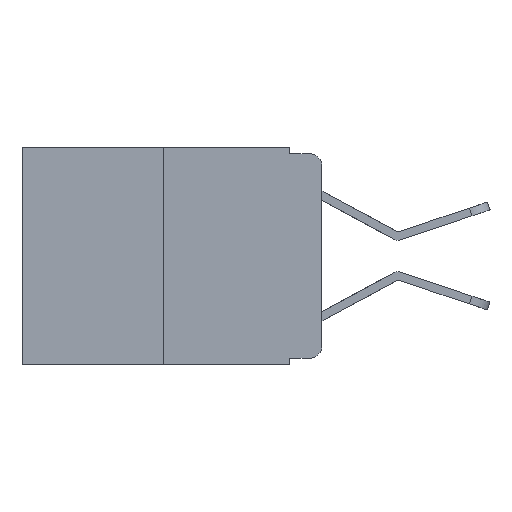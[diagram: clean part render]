
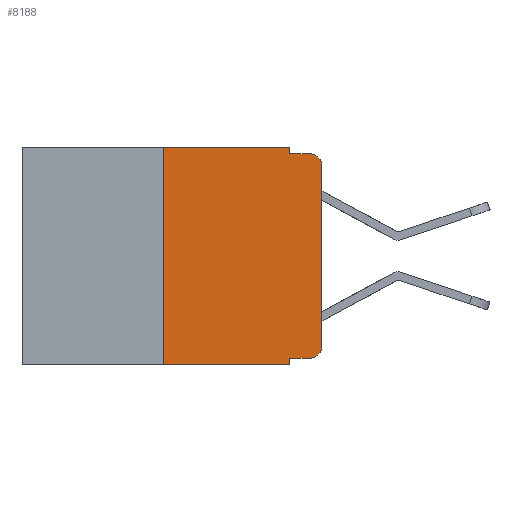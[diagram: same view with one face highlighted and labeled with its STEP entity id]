
A CAD part, left-side view. The second image highlights one B-rep face of the part: STEP entity #8188.
In plain terms, the highlighted planar face has unit normal (-1, 0, 0).
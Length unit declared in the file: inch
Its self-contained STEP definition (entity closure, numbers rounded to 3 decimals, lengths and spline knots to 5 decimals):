
#37 = EDGE_CURVE ( 'NONE', #5727, #10715, #5399, .T. ) ;
#81 = DIRECTION ( 'NONE',  ( 0., -1., 0. ) ) ;
#416 = CARTESIAN_POINT ( 'NONE',  ( 0., 0.02, -0.01 ) ) ;
#569 = CARTESIAN_POINT ( 'NONE',  ( 0., 0., -0.313 ) ) ;
#613 = DIRECTION ( 'NONE',  ( 0., 0., -1. ) ) ;
#999 = ORIENTED_EDGE ( 'NONE', *, *, #1486, .F. ) ;
#1174 = CARTESIAN_POINT ( 'NONE',  ( 0., 0.051, 0. ) ) ;
#1313 = VECTOR ( 'NONE', #13324, 39.37008 ) ;
#1486 = EDGE_CURVE ( 'NONE', #10284, #11984, #14424, .T. ) ;
#1920 = VERTEX_POINT ( 'NONE', #12047 ) ;
#1991 = DIRECTION ( 'NONE',  ( 1., 0., 0. ) ) ;
#2308 = EDGE_CURVE ( 'NONE', #11984, #10111, #4769, .T. ) ;
#2555 = VECTOR ( 'NONE', #4273, 39.37008 ) ;
#2671 = DIRECTION ( 'NONE',  ( 0., -1., 0. ) ) ;
#2691 = CIRCLE ( 'NONE', #7017, 0.02 ) ;
#3013 = VECTOR ( 'NONE', #9646, 39.37008 ) ;
#3077 = VECTOR ( 'NONE', #2671, 39.37008 ) ;
#3184 = LINE ( 'NONE', #7799, #3722 ) ;
#3427 = ORIENTED_EDGE ( 'NONE', *, *, #11608, .T. ) ;
#3722 = VECTOR ( 'NONE', #81, 39.37008 ) ;
#3765 = ORIENTED_EDGE ( 'NONE', *, *, #12278, .F. ) ;
#3883 = CARTESIAN_POINT ( 'NONE',  ( 0., 0.25, 0. ) ) ;
#4033 = ORIENTED_EDGE ( 'NONE', *, *, #2308, .F. ) ;
#4186 = ORIENTED_EDGE ( 'NONE', *, *, #12717, .F. ) ;
#4271 = CARTESIAN_POINT ( 'NONE',  ( 0., 0.25, 0. ) ) ;
#4273 = DIRECTION ( 'NONE',  ( 0., 0., -1. ) ) ;
#4377 = ORIENTED_EDGE ( 'NONE', *, *, #7946, .T. ) ;
#4607 = VERTEX_POINT ( 'NONE', #11918 ) ;
#4769 = LINE ( 'NONE', #9403, #3077 ) ;
#5012 = VECTOR ( 'NONE', #12851, 39.37008 ) ;
#5063 = DIRECTION ( 'NONE',  ( -1., 0., 0. ) ) ;
#5078 = LINE ( 'NONE', #3883, #3013 ) ;
#5274 = CARTESIAN_POINT ( 'NONE',  ( 0., 0., -0.03 ) ) ;
#5308 = LINE ( 'NONE', #11133, #1313 ) ;
#5399 = LINE ( 'NONE', #12344, #5012 ) ;
#5539 = CARTESIAN_POINT ( 'NONE',  ( 0., 0.473, 0. ) ) ;
#5700 = CIRCLE ( 'NONE', #13659, 0.02 ) ;
#5727 = VERTEX_POINT ( 'NONE', #569 ) ;
#6055 = CARTESIAN_POINT ( 'NONE',  ( 0., 0.25, -0.343 ) ) ;
#6186 = AXIS2_PLACEMENT_3D ( 'NONE', #5539, #1991, #11215 ) ;
#6683 = ORIENTED_EDGE ( 'NONE', *, *, #37, .T. ) ;
#6696 = DIRECTION ( 'NONE',  ( 0., 0., -1. ) ) ;
#6735 = VERTEX_POINT ( 'NONE', #4271 ) ;
#6973 = ORIENTED_EDGE ( 'NONE', *, *, #9064, .T. ) ;
#7017 = AXIS2_PLACEMENT_3D ( 'NONE', #9837, #5063, #613 ) ;
#7126 = VECTOR ( 'NONE', #9955, 39.37008 ) ;
#7762 = FACE_OUTER_BOUND ( 'NONE', #10482, .T. ) ;
#7799 = CARTESIAN_POINT ( 'NONE',  ( 0., 0.473, -0.343 ) ) ;
#7946 = EDGE_CURVE ( 'NONE', #10715, #10111, #2691, .T. ) ;
#7966 = CARTESIAN_POINT ( 'NONE',  ( 0., 0.02, -0.313 ) ) ;
#8121 = VECTOR ( 'NONE', #6696, 39.37008 ) ;
#8188 = ADVANCED_FACE ( 'NONE', ( #7762 ), #12337, .F. ) ;
#8702 = CARTESIAN_POINT ( 'NONE',  ( 0., 0.473, 0. ) ) ;
#8847 = VERTEX_POINT ( 'NONE', #6055 ) ;
#9012 = CARTESIAN_POINT ( 'NONE',  ( 0., 0.051, 0. ) ) ;
#9064 = EDGE_CURVE ( 'NONE', #8847, #4607, #3184, .T. ) ;
#9403 = CARTESIAN_POINT ( 'NONE',  ( 0., 0.051, -0.01 ) ) ;
#9457 = VERTEX_POINT ( 'NONE', #9904 ) ;
#9646 = DIRECTION ( 'NONE',  ( 0., 0., 1. ) ) ;
#9837 = CARTESIAN_POINT ( 'NONE',  ( 0., 0.02, -0.03 ) ) ;
#9904 = CARTESIAN_POINT ( 'NONE',  ( 0., 0.051, -0.333 ) ) ;
#9955 = DIRECTION ( 'NONE',  ( 0., -1., 0. ) ) ;
#10111 = VERTEX_POINT ( 'NONE', #416 ) ;
#10284 = VERTEX_POINT ( 'NONE', #9012 ) ;
#10429 = ORIENTED_EDGE ( 'NONE', *, *, #13729, .T. ) ;
#10482 = EDGE_LOOP ( 'NONE', ( #6683, #4377, #4033, #999, #4186, #3765, #6973, #13296, #3427, #10429 ) ) ;
#10715 = VERTEX_POINT ( 'NONE', #5274 ) ;
#10742 = CARTESIAN_POINT ( 'NONE',  ( 0., 0.051, -0.01 ) ) ;
#11016 = LINE ( 'NONE', #8702, #7126 ) ;
#11133 = CARTESIAN_POINT ( 'NONE',  ( 0., 0.051, -0.333 ) ) ;
#11187 = DIRECTION ( 'NONE',  ( 0., 0., -1. ) ) ;
#11215 = DIRECTION ( 'NONE',  ( 0., 0., -1. ) ) ;
#11608 = EDGE_CURVE ( 'NONE', #9457, #1920, #5308, .T. ) ;
#11918 = CARTESIAN_POINT ( 'NONE',  ( 0., 0.051, -0.343 ) ) ;
#11984 = VERTEX_POINT ( 'NONE', #10742 ) ;
#12047 = CARTESIAN_POINT ( 'NONE',  ( 0., 0.02, -0.333 ) ) ;
#12278 = EDGE_CURVE ( 'NONE', #8847, #6735, #5078, .T. ) ;
#12283 = CARTESIAN_POINT ( 'NONE',  ( 0., 0.051, 0. ) ) ;
#12337 = PLANE ( 'NONE',  #6186 ) ;
#12344 = CARTESIAN_POINT ( 'NONE',  ( 0., 0., 0. ) ) ;
#12717 = EDGE_CURVE ( 'NONE', #6735, #10284, #11016, .T. ) ;
#12851 = DIRECTION ( 'NONE',  ( 0., 0., 1. ) ) ;
#13260 = EDGE_CURVE ( 'NONE', #9457, #4607, #14768, .T. ) ;
#13296 = ORIENTED_EDGE ( 'NONE', *, *, #13260, .F. ) ;
#13324 = DIRECTION ( 'NONE',  ( 0., -1., 0. ) ) ;
#13659 = AXIS2_PLACEMENT_3D ( 'NONE', #7966, #13682, #11187 ) ;
#13682 = DIRECTION ( 'NONE',  ( -1., 0., 0. ) ) ;
#13729 = EDGE_CURVE ( 'NONE', #1920, #5727, #5700, .T. ) ;
#14424 = LINE ( 'NONE', #12283, #2555 ) ;
#14768 = LINE ( 'NONE', #1174, #8121 ) ;
